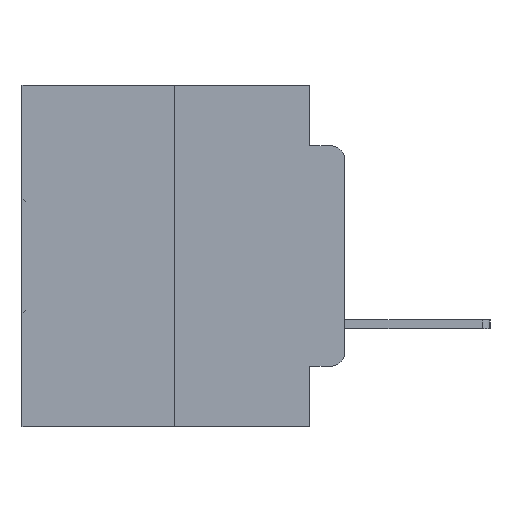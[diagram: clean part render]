
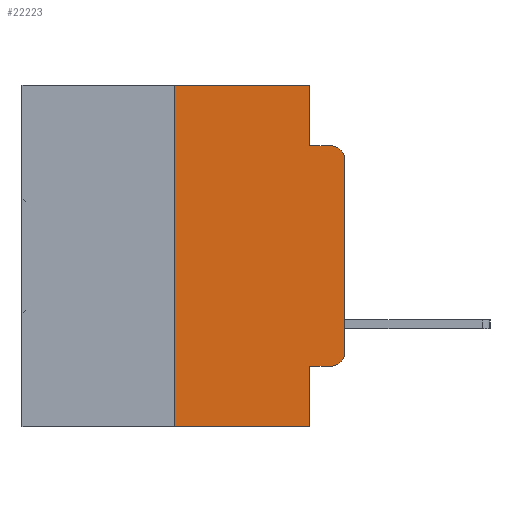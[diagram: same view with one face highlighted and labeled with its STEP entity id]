
A CAD part, left-side view. The second image highlights one B-rep face of the part: STEP entity #22223.
In plain terms, the highlighted planar face has unit normal (-1, 0, 0).
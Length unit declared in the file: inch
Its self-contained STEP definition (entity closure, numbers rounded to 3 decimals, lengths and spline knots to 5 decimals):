
#622 = CARTESIAN_POINT ( 'NONE',  ( 0., 0.25, 0. ) ) ;
#1355 = VECTOR ( 'NONE', #16594, 39.37008 ) ;
#2080 = DIRECTION ( 'NONE',  ( 0., 0., -1. ) ) ;
#2257 = CARTESIAN_POINT ( 'NONE',  ( 0., 0.051, -0.5 ) ) ;
#2382 = CARTESIAN_POINT ( 'NONE',  ( 0., 0.051, -0.4115 ) ) ;
#2759 = CARTESIAN_POINT ( 'NONE',  ( 0., 0.25, -0.5 ) ) ;
#2825 = CARTESIAN_POINT ( 'NONE',  ( 0., 0., 0. ) ) ;
#3275 = ORIENTED_EDGE ( 'NONE', *, *, #25850, .F. ) ;
#3406 = EDGE_CURVE ( 'NONE', #19735, #9299, #22029, .T. ) ;
#3673 = VERTEX_POINT ( 'NONE', #2759 ) ;
#4163 = DIRECTION ( 'NONE',  ( -1., 0., 0. ) ) ;
#4579 = EDGE_CURVE ( 'NONE', #25545, #5170, #19040, .T. ) ;
#4814 = DIRECTION ( 'NONE',  ( 0., -1., 0. ) ) ;
#4960 = VERTEX_POINT ( 'NONE', #22139 ) ;
#5170 = VERTEX_POINT ( 'NONE', #22928 ) ;
#5260 = DIRECTION ( 'NONE',  ( 0., 0., 1. ) ) ;
#5345 = DIRECTION ( 'NONE',  ( 0., 0., 1. ) ) ;
#5528 = CARTESIAN_POINT ( 'NONE',  ( 0., 0.051, 0. ) ) ;
#5783 = DIRECTION ( 'NONE',  ( -1., 0., 0. ) ) ;
#6198 = EDGE_CURVE ( 'NONE', #11595, #25545, #29494, .T. ) ;
#6333 = DIRECTION ( 'NONE',  ( 0., -1., 0. ) ) ;
#6671 = ORIENTED_EDGE ( 'NONE', *, *, #4579, .T. ) ;
#7798 = LINE ( 'NONE', #30635, #1355 ) ;
#8180 = ORIENTED_EDGE ( 'NONE', *, *, #3406, .F. ) ;
#9181 = VECTOR ( 'NONE', #5260, 39.37008 ) ;
#9299 = VERTEX_POINT ( 'NONE', #30294 ) ;
#10211 = VECTOR ( 'NONE', #24481, 39.37008 ) ;
#10648 = EDGE_CURVE ( 'NONE', #3673, #22164, #7798, .T. ) ;
#11456 = AXIS2_PLACEMENT_3D ( 'NONE', #18440, #4163, #20801 ) ;
#11595 = VERTEX_POINT ( 'NONE', #13335 ) ;
#11873 = CARTESIAN_POINT ( 'NONE',  ( 0., 0.051, -0.4115 ) ) ;
#11907 = CIRCLE ( 'NONE', #12351, 0.02 ) ;
#11940 = ORIENTED_EDGE ( 'NONE', *, *, #17942, .T. ) ;
#12351 = AXIS2_PLACEMENT_3D ( 'NONE', #19990, #5783, #22347 ) ;
#12478 = CARTESIAN_POINT ( 'NONE',  ( 0., 0.25, 0. ) ) ;
#13335 = CARTESIAN_POINT ( 'NONE',  ( 0., 0., -0.3915 ) ) ;
#13531 = VECTOR ( 'NONE', #6333, 39.37008 ) ;
#13694 = LINE ( 'NONE', #2382, #19181 ) ;
#13800 = CARTESIAN_POINT ( 'NONE',  ( 0., 0.473, 0. ) ) ;
#13805 = ORIENTED_EDGE ( 'NONE', *, *, #29006, .F. ) ;
#14480 = DIRECTION ( 'NONE',  ( 0., 0., -1. ) ) ;
#14650 = FACE_OUTER_BOUND ( 'NONE', #17913, .T. ) ;
#14870 = VECTOR ( 'NONE', #2080, 39.37008 ) ;
#15578 = LINE ( 'NONE', #30495, #14870 ) ;
#16594 = DIRECTION ( 'NONE',  ( 0., -1., 0. ) ) ;
#17488 = ORIENTED_EDGE ( 'NONE', *, *, #21091, .F. ) ;
#17913 = EDGE_LOOP ( 'NONE', ( #30323, #6671, #13805, #20042, #8180, #3275, #22260, #17488, #29262, #11940 ) ) ;
#17942 = EDGE_CURVE ( 'NONE', #26120, #11595, #11907, .T. ) ;
#18176 = CARTESIAN_POINT ( 'NONE',  ( 0., 0.051, -0.0885 ) ) ;
#18440 = CARTESIAN_POINT ( 'NONE',  ( 0., 0.02, -0.1085 ) ) ;
#19040 = CIRCLE ( 'NONE', #11456, 0.02 ) ;
#19181 = VECTOR ( 'NONE', #4814, 39.37008 ) ;
#19532 = EDGE_CURVE ( 'NONE', #27486, #26120, #13694, .T. ) ;
#19735 = VERTEX_POINT ( 'NONE', #622 ) ;
#19779 = LINE ( 'NONE', #18176, #13531 ) ;
#19990 = CARTESIAN_POINT ( 'NONE',  ( 0., 0.02, -0.3915 ) ) ;
#20042 = ORIENTED_EDGE ( 'NONE', *, *, #27433, .F. ) ;
#20701 = CARTESIAN_POINT ( 'NONE',  ( 0., 0., -0.1085 ) ) ;
#20801 = DIRECTION ( 'NONE',  ( 0., 0., -1. ) ) ;
#21091 = EDGE_CURVE ( 'NONE', #27486, #22164, #29752, .T. ) ;
#21286 = VECTOR ( 'NONE', #25515, 39.37008 ) ;
#22029 = LINE ( 'NONE', #13800, #21286 ) ;
#22139 = CARTESIAN_POINT ( 'NONE',  ( 0., 0.051, -0.0885 ) ) ;
#22164 = VERTEX_POINT ( 'NONE', #2257 ) ;
#22223 = ADVANCED_FACE ( 'NONE', ( #14650 ), #23786, .F. ) ;
#22260 = ORIENTED_EDGE ( 'NONE', *, *, #10648, .T. ) ;
#22272 = LINE ( 'NONE', #12478, #23749 ) ;
#22347 = DIRECTION ( 'NONE',  ( 0., 0., -1. ) ) ;
#22928 = CARTESIAN_POINT ( 'NONE',  ( 0., 0.02, -0.0885 ) ) ;
#23749 = VECTOR ( 'NONE', #5345, 39.37008 ) ;
#23786 = PLANE ( 'NONE',  #24673 ) ;
#24481 = DIRECTION ( 'NONE',  ( 0., 0., -1. ) ) ;
#24673 = AXIS2_PLACEMENT_3D ( 'NONE', #26189, #28549, #14480 ) ;
#25515 = DIRECTION ( 'NONE',  ( 0., -1., 0. ) ) ;
#25545 = VERTEX_POINT ( 'NONE', #20701 ) ;
#25850 = EDGE_CURVE ( 'NONE', #3673, #19735, #22272, .T. ) ;
#26120 = VERTEX_POINT ( 'NONE', #29916 ) ;
#26189 = CARTESIAN_POINT ( 'NONE',  ( 0., 0.473, 0. ) ) ;
#27433 = EDGE_CURVE ( 'NONE', #9299, #4960, #15578, .T. ) ;
#27486 = VERTEX_POINT ( 'NONE', #11873 ) ;
#28549 = DIRECTION ( 'NONE',  ( 1., 0., 0. ) ) ;
#29006 = EDGE_CURVE ( 'NONE', #4960, #5170, #19779, .T. ) ;
#29262 = ORIENTED_EDGE ( 'NONE', *, *, #19532, .T. ) ;
#29494 = LINE ( 'NONE', #2825, #9181 ) ;
#29752 = LINE ( 'NONE', #5528, #10211 ) ;
#29916 = CARTESIAN_POINT ( 'NONE',  ( 0., 0.02, -0.4115 ) ) ;
#30294 = CARTESIAN_POINT ( 'NONE',  ( 0., 0.051, 0. ) ) ;
#30323 = ORIENTED_EDGE ( 'NONE', *, *, #6198, .T. ) ;
#30495 = CARTESIAN_POINT ( 'NONE',  ( 0., 0.051, 0. ) ) ;
#30635 = CARTESIAN_POINT ( 'NONE',  ( 0., 0.473, -0.5 ) ) ;
